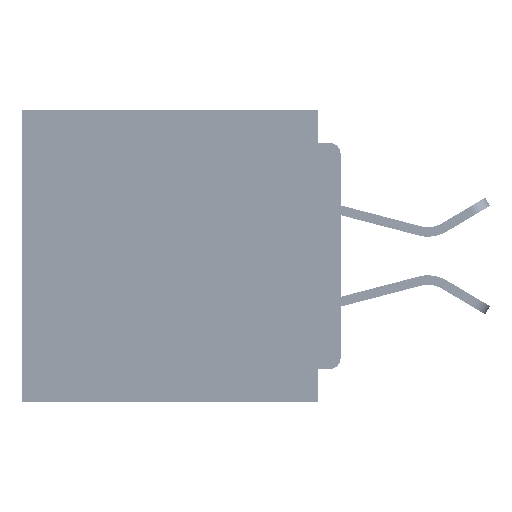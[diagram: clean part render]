
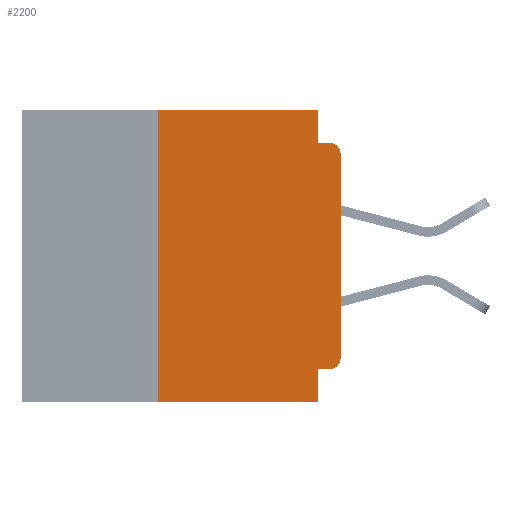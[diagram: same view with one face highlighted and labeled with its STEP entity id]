
A CAD part, left-side view. The second image highlights one B-rep face of the part: STEP entity #2200.
In plain terms, the highlighted planar face has unit normal (-1, 0, 0).
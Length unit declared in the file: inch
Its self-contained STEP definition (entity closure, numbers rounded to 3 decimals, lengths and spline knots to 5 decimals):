
#480 = DIRECTION ( 'NONE',  ( 0., 0., -1. ) ) ;
#1059 = AXIS2_PLACEMENT_3D ( 'NONE', #39597, #12132, #44147 ) ;
#2200 = ADVANCED_FACE ( 'NONE', ( #41040 ), #11123, .F. ) ;
#2418 = LINE ( 'NONE', #9438, #49669 ) ;
#3823 = VERTEX_POINT ( 'NONE', #7735 ) ;
#4068 = CARTESIAN_POINT ( 'NONE',  ( 0., 0.015, -0.34 ) ) ;
#4428 = CARTESIAN_POINT ( 'NONE',  ( 0., 0.031, -0.045 ) ) ;
#4860 = EDGE_CURVE ( 'NONE', #12098, #51155, #40136, .T. ) ;
#4925 = ORIENTED_EDGE ( 'NONE', *, *, #11774, .T. ) ;
#5077 = CARTESIAN_POINT ( 'NONE',  ( 0., 0.031, 0. ) ) ;
#5107 = VECTOR ( 'NONE', #20448, 39.37008 ) ;
#5187 = LINE ( 'NONE', #14974, #52403 ) ;
#5328 = EDGE_CURVE ( 'NONE', #43581, #33131, #38669, .T. ) ;
#5380 = DIRECTION ( 'NONE',  ( 0., 0., 1. ) ) ;
#6424 = DIRECTION ( 'NONE',  ( 0., 0., -1. ) ) ;
#7735 = CARTESIAN_POINT ( 'NONE',  ( 0., 0.031, 0. ) ) ;
#8412 = VERTEX_POINT ( 'NONE', #49089 ) ;
#8620 = EDGE_CURVE ( 'NONE', #33131, #3823, #2418, .T. ) ;
#8662 = DIRECTION ( 'NONE',  ( 0., 0., -1. ) ) ;
#8903 = ORIENTED_EDGE ( 'NONE', *, *, #57175, .T. ) ;
#9438 = CARTESIAN_POINT ( 'NONE',  ( 0., 0.437, 0. ) ) ;
#9984 = EDGE_CURVE ( 'NONE', #8412, #12098, #11517, .T. ) ;
#10087 = DIRECTION ( 'NONE',  ( 0., 0., -1. ) ) ;
#10144 = AXIS2_PLACEMENT_3D ( 'NONE', #10983, #11108, #10087 ) ;
#10983 = CARTESIAN_POINT ( 'NONE',  ( 0., 0.437, 0. ) ) ;
#11108 = DIRECTION ( 'NONE',  ( 1., 0., 0. ) ) ;
#11123 = PLANE ( 'NONE',  #10144 ) ;
#11453 = CARTESIAN_POINT ( 'NONE',  ( 0., 0.015, -0.045 ) ) ;
#11517 = LINE ( 'NONE', #54228, #58761 ) ;
#11774 = EDGE_CURVE ( 'NONE', #8412, #43065, #32706, .T. ) ;
#12098 = VERTEX_POINT ( 'NONE', #56612 ) ;
#12132 = DIRECTION ( 'NONE',  ( -1., 0., 0. ) ) ;
#12693 = ORIENTED_EDGE ( 'NONE', *, *, #8620, .F. ) ;
#14011 = CARTESIAN_POINT ( 'NONE',  ( 0., 0.031, -0.4 ) ) ;
#14670 = EDGE_CURVE ( 'NONE', #28844, #26210, #5187, .T. ) ;
#14974 = CARTESIAN_POINT ( 'NONE',  ( 0., 0., -0.045 ) ) ;
#19783 = EDGE_CURVE ( 'NONE', #3823, #28844, #30249, .T. ) ;
#20436 = CARTESIAN_POINT ( 'NONE',  ( 0., 0., -0.34 ) ) ;
#20448 = DIRECTION ( 'NONE',  ( 0., 0., 1. ) ) ;
#20455 = VECTOR ( 'NONE', #36306, 39.37008 ) ;
#21987 = CARTESIAN_POINT ( 'NONE',  ( 0., 0., -0.06 ) ) ;
#22064 = ORIENTED_EDGE ( 'NONE', *, *, #5328, .F. ) ;
#22182 = CARTESIAN_POINT ( 'NONE',  ( 0., 0.25, 0. ) ) ;
#25980 = AXIS2_PLACEMENT_3D ( 'NONE', #4068, #36131, #8662 ) ;
#26210 = VERTEX_POINT ( 'NONE', #11453 ) ;
#27895 = DIRECTION ( 'NONE',  ( 0., -1., 0. ) ) ;
#28007 = VECTOR ( 'NONE', #6424, 39.37008 ) ;
#28844 = VERTEX_POINT ( 'NONE', #4428 ) ;
#29282 = CARTESIAN_POINT ( 'NONE',  ( 0., 0.031, -0.4 ) ) ;
#30249 = LINE ( 'NONE', #5077, #42367 ) ;
#31686 = CARTESIAN_POINT ( 'NONE',  ( 0., 0.437, -0.4 ) ) ;
#32706 = CIRCLE ( 'NONE', #25980, 0.015 ) ;
#32821 = CARTESIAN_POINT ( 'NONE',  ( 0., 0.25, -0.4 ) ) ;
#33010 = ORIENTED_EDGE ( 'NONE', *, *, #14670, .F. ) ;
#33131 = VERTEX_POINT ( 'NONE', #22182 ) ;
#34590 = ORIENTED_EDGE ( 'NONE', *, *, #40994, .T. ) ;
#36131 = DIRECTION ( 'NONE',  ( -1., 0., 0. ) ) ;
#36306 = DIRECTION ( 'NONE',  ( 0., -1., 0. ) ) ;
#36485 = EDGE_LOOP ( 'NONE', ( #34590, #8903, #33010, #56893, #12693, #22064, #39731, #49634, #40578, #4925 ) ) ;
#38003 = CARTESIAN_POINT ( 'NONE',  ( 0., 0.25, -0.4 ) ) ;
#38669 = LINE ( 'NONE', #32821, #49383 ) ;
#39597 = CARTESIAN_POINT ( 'NONE',  ( 0., 0.015, -0.06 ) ) ;
#39731 = ORIENTED_EDGE ( 'NONE', *, *, #44911, .T. ) ;
#40136 = LINE ( 'NONE', #29282, #28007 ) ;
#40191 = LINE ( 'NONE', #43411, #5107 ) ;
#40578 = ORIENTED_EDGE ( 'NONE', *, *, #9984, .F. ) ;
#40994 = EDGE_CURVE ( 'NONE', #43065, #43785, #40191, .T. ) ;
#41040 = FACE_OUTER_BOUND ( 'NONE', #36485, .T. ) ;
#42367 = VECTOR ( 'NONE', #480, 39.37008 ) ;
#43065 = VERTEX_POINT ( 'NONE', #20436 ) ;
#43411 = CARTESIAN_POINT ( 'NONE',  ( 0., 0., 0. ) ) ;
#43581 = VERTEX_POINT ( 'NONE', #38003 ) ;
#43785 = VERTEX_POINT ( 'NONE', #21987 ) ;
#44147 = DIRECTION ( 'NONE',  ( 0., 0., -1. ) ) ;
#44911 = EDGE_CURVE ( 'NONE', #43581, #51155, #52630, .T. ) ;
#49089 = CARTESIAN_POINT ( 'NONE',  ( 0., 0.015, -0.355 ) ) ;
#49383 = VECTOR ( 'NONE', #5380, 39.37008 ) ;
#49634 = ORIENTED_EDGE ( 'NONE', *, *, #4860, .F. ) ;
#49669 = VECTOR ( 'NONE', #27895, 39.37008 ) ;
#49683 = DIRECTION ( 'NONE',  ( 0., 1., 0. ) ) ;
#51081 = CIRCLE ( 'NONE', #1059, 0.015 ) ;
#51155 = VERTEX_POINT ( 'NONE', #14011 ) ;
#52403 = VECTOR ( 'NONE', #56200, 39.37008 ) ;
#52630 = LINE ( 'NONE', #31686, #20455 ) ;
#54228 = CARTESIAN_POINT ( 'NONE',  ( 0., 0., -0.355 ) ) ;
#56200 = DIRECTION ( 'NONE',  ( 0., -1., 0. ) ) ;
#56612 = CARTESIAN_POINT ( 'NONE',  ( 0., 0.031, -0.355 ) ) ;
#56893 = ORIENTED_EDGE ( 'NONE', *, *, #19783, .F. ) ;
#57175 = EDGE_CURVE ( 'NONE', #43785, #26210, #51081, .T. ) ;
#58761 = VECTOR ( 'NONE', #49683, 39.37008 ) ;
